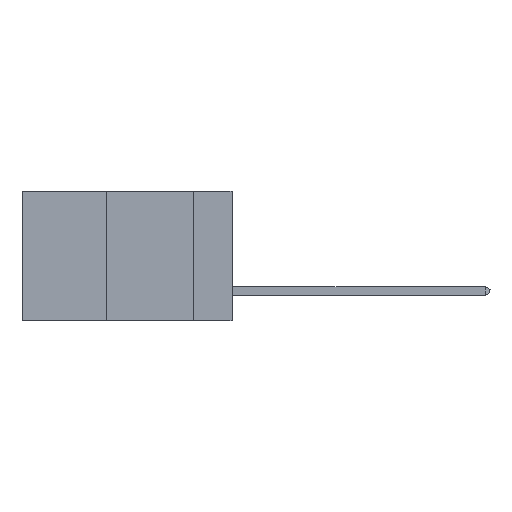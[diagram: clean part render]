
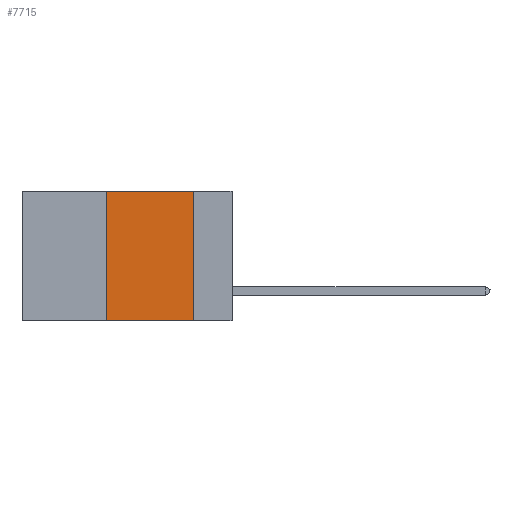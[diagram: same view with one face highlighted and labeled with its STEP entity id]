
A CAD part, left-side view. The second image highlights one B-rep face of the part: STEP entity #7715.
In plain terms, the highlighted planar face has unit normal (-1, 0, 0).
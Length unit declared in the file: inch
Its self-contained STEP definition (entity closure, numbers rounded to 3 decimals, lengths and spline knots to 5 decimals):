
#2606 = EDGE_CURVE ( 'NONE', #8668, #20492, #18627, .T. ) ;
#2813 = FACE_OUTER_BOUND ( 'NONE', #25739, .T. ) ;
#3637 = VECTOR ( 'NONE', #13049, 39.37008 ) ;
#4056 = PLANE ( 'NONE',  #22174 ) ;
#6311 = CARTESIAN_POINT ( 'NONE',  ( 0., 0.36, -0.37 ) ) ;
#7715 = ADVANCED_FACE ( 'NONE', ( #2813 ), #4056, .F. ) ;
#8668 = VERTEX_POINT ( 'NONE', #31152 ) ;
#9213 = ORIENTED_EDGE ( 'NONE', *, *, #2606, .F. ) ;
#9682 = DIRECTION ( 'NONE',  ( 0., -1., 0. ) ) ;
#10772 = DIRECTION ( 'NONE',  ( 0., 0., -1. ) ) ;
#11376 = CARTESIAN_POINT ( 'NONE',  ( 0., 0.6, 0. ) ) ;
#13049 = DIRECTION ( 'NONE',  ( 0., 0., -1. ) ) ;
#13565 = CARTESIAN_POINT ( 'NONE',  ( 0., 0.36, 0. ) ) ;
#15038 = CARTESIAN_POINT ( 'NONE',  ( 0., 0.11, 0. ) ) ;
#15157 = EDGE_CURVE ( 'NONE', #42544, #8668, #43652, .T. ) ;
#16929 = CARTESIAN_POINT ( 'NONE',  ( 0., 0.6, -0.37 ) ) ;
#17548 = ORIENTED_EDGE ( 'NONE', *, *, #15157, .F. ) ;
#17685 = EDGE_CURVE ( 'NONE', #20492, #25215, #41233, .T. ) ;
#18627 = LINE ( 'NONE', #11376, #44008 ) ;
#19025 = CARTESIAN_POINT ( 'NONE',  ( 0., 0.6, 0. ) ) ;
#20492 = VERTEX_POINT ( 'NONE', #15038 ) ;
#20511 = VECTOR ( 'NONE', #38300, 39.37008 ) ;
#21430 = VECTOR ( 'NONE', #9682, 39.37008 ) ;
#22174 = AXIS2_PLACEMENT_3D ( 'NONE', #19025, #30894, #10772 ) ;
#23552 = CARTESIAN_POINT ( 'NONE',  ( 0., 0.11, 0. ) ) ;
#25215 = VERTEX_POINT ( 'NONE', #34216 ) ;
#25739 = EDGE_LOOP ( 'NONE', ( #34867, #9213, #17548, #43539 ) ) ;
#30894 = DIRECTION ( 'NONE',  ( 1., 0., 0. ) ) ;
#30925 = LINE ( 'NONE', #16929, #21430 ) ;
#31152 = CARTESIAN_POINT ( 'NONE',  ( 0., 0.36, 0. ) ) ;
#34216 = CARTESIAN_POINT ( 'NONE',  ( 0., 0.11, -0.37 ) ) ;
#34867 = ORIENTED_EDGE ( 'NONE', *, *, #17685, .F. ) ;
#35926 = DIRECTION ( 'NONE',  ( 0., -1., 0. ) ) ;
#38300 = DIRECTION ( 'NONE',  ( 0., 0., 1. ) ) ;
#41233 = LINE ( 'NONE', #23552, #3637 ) ;
#42544 = VERTEX_POINT ( 'NONE', #6311 ) ;
#43467 = EDGE_CURVE ( 'NONE', #42544, #25215, #30925, .T. ) ;
#43539 = ORIENTED_EDGE ( 'NONE', *, *, #43467, .T. ) ;
#43652 = LINE ( 'NONE', #13565, #20511 ) ;
#44008 = VECTOR ( 'NONE', #35926, 39.37008 ) ;
